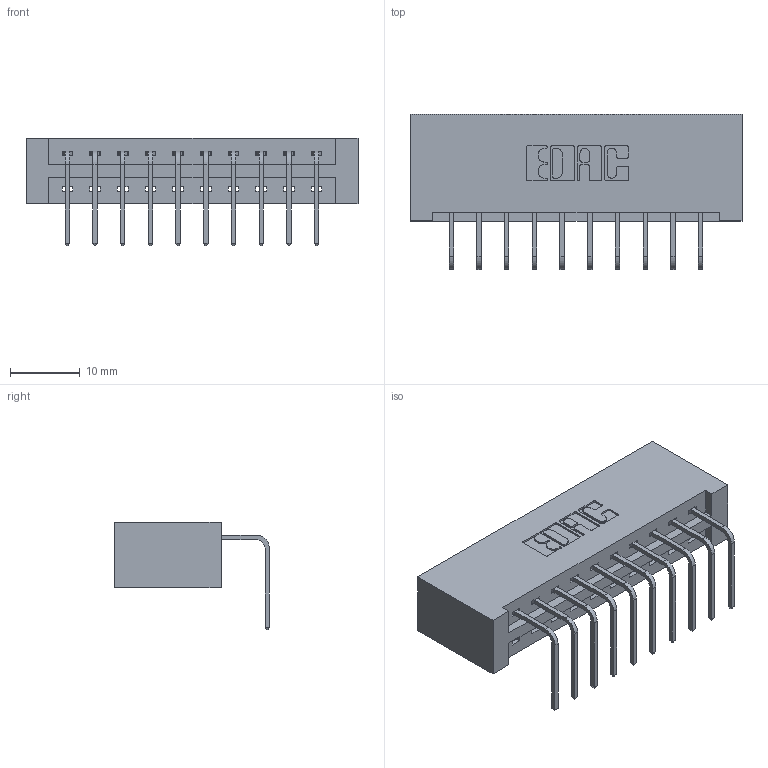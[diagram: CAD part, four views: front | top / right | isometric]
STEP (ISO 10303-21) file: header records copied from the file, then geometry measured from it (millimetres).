
FILE_DESCRIPTION (( 'STEP AP203' ), '1' );
FILE_NAME ('387-010-558-101.STEP', '2018-09-10T07:31:59', ( '' ), ( '' ), 'SwSTEP 2.0', 'SolidWorks 2016', '' );
FILE_SCHEMA (( 'CONFIG_CONTROL_DESIGN' ));
Length unit declared in the file: inch
Products named in the file (3): 337 Part_No Mounting Lugs; 345-292-001_558 Tail - 2; 387-010-558-101
Assembly tree (11 placements, depth 2):
  387-010-558-101
    337 Part_No Mounting Lugs
    345-292-001_558 Tail - 2  x10
Bounding box: 47.5 x 22.17 x 15.37 mm (x, y, z)
Volume: 5308.2 mm3; surface area: 5493.8 mm2
Topology: 11 solids, 11 shells, 746 faces, 2227 edges, 1470 vertices
Faces by surface type: plane 546, cylinder 200
Entity records: 11379 total; most frequent: CARTESIAN_POINT 1988, ORIENTED_EDGE 1934, DIRECTION 1731, EDGE_CURVE 967, VECTOR 847, LINE 847, VERTEX_POINT 642, AXIS2_PLACEMENT_3D 442
